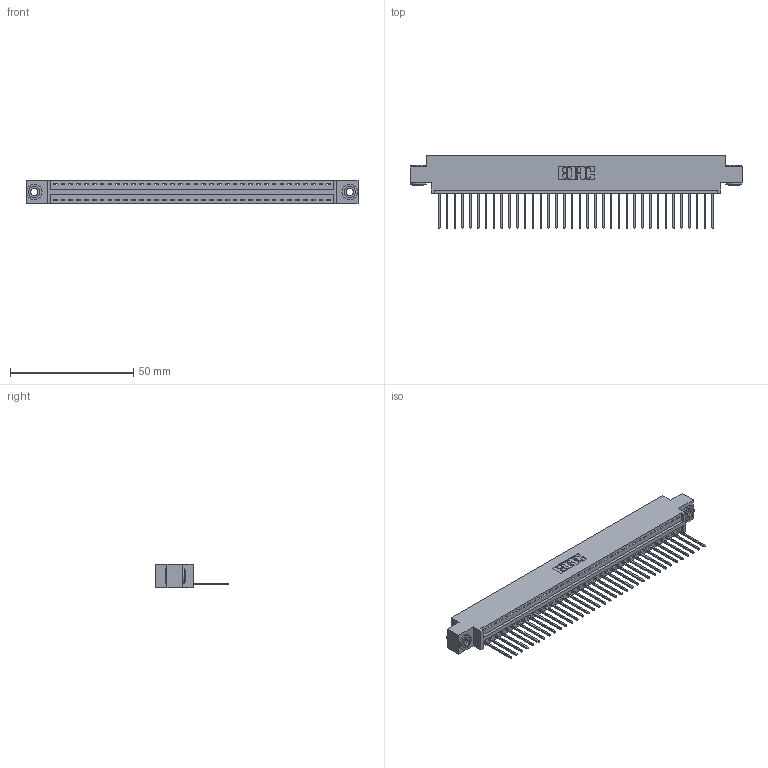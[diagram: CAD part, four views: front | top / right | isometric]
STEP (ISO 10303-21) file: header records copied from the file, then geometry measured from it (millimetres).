
FILE_DESCRIPTION (( 'STEP AP203' ), '1' );
FILE_NAME ('346-036-540-603.STEP', '2022-05-07T01:09:57', ( '' ), ( '' ), 'SwSTEP 2.0', 'SolidWorks 2020', '' );
FILE_SCHEMA (( 'CONFIG_CONTROL_DESIGN' ));
Length unit declared in the file: inch
Products named in the file (4): 345-292-001_345-293-140; 346 Part_0.170 Offset - 0.156 Dia-TH; 345-250-002_345-250-002-102; 346-036-540-603
Assembly tree (39 placements, depth 2):
  346-036-540-603
    346 Part_0.170 Offset - 0.156 Dia-TH
    345-292-001_345-293-140  x36
    345-250-002_345-250-002-102  x2
Bounding box: 134.87 x 29.46 x 9.4 mm (x, y, z)
Volume: 12764.5 mm3; surface area: 16657 mm2
Topology: 39 solids, 39 shells, 2266 faces, 6789 edges, 4474 vertices
Faces by surface type: plane 1544, cylinder 714, cone 8
Entity records: 24366 total; most frequent: CARTESIAN_POINT 4161, ORIENTED_EDGE 4122, DIRECTION 3707, EDGE_CURVE 2061, VECTOR 1761, LINE 1761, VERTEX_POINT 1370, AXIS2_PLACEMENT_3D 973
